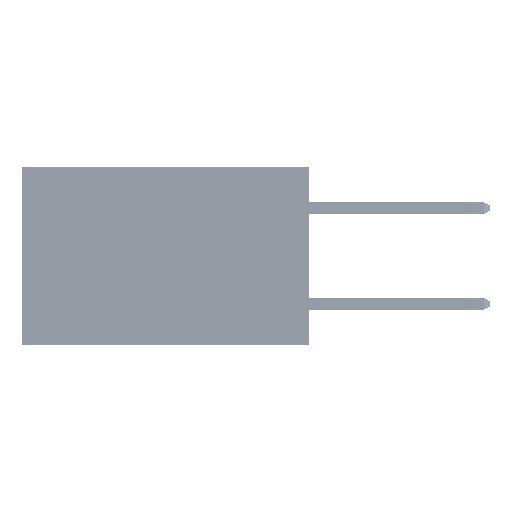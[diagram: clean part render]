
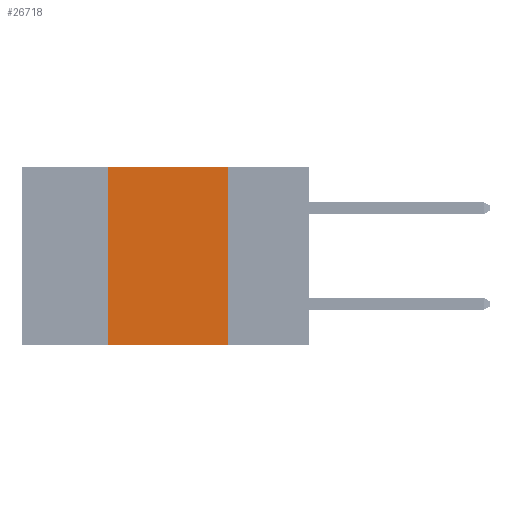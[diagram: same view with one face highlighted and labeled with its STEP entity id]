
A CAD part, left-side view. The second image highlights one B-rep face of the part: STEP entity #26718.
In plain terms, the highlighted planar face has unit normal (-1, 0, 0).
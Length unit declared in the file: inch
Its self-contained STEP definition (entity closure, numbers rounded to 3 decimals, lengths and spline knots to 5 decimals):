
#3771 = LINE ( 'NONE', #43292, #22693 ) ;
#4714 = ORIENTED_EDGE ( 'NONE', *, *, #41094, .F. ) ;
#6899 = CARTESIAN_POINT ( 'NONE',  ( 0., 0.6, 0. ) ) ;
#7054 = CARTESIAN_POINT ( 'NONE',  ( 0., 0.42, 0. ) ) ;
#7142 = EDGE_CURVE ( 'NONE', #38071, #16841, #40286, .T. ) ;
#8549 = LINE ( 'NONE', #7054, #18043 ) ;
#9423 = EDGE_CURVE ( 'NONE', #12495, #20548, #3771, .T. ) ;
#10263 = EDGE_CURVE ( 'NONE', #16841, #20548, #38269, .T. ) ;
#10936 = DIRECTION ( 'NONE',  ( 0., 0., -1. ) ) ;
#12495 = VERTEX_POINT ( 'NONE', #46830 ) ;
#15888 = EDGE_LOOP ( 'NONE', ( #47337, #34877, #4714, #20525 ) ) ;
#16715 = CARTESIAN_POINT ( 'NONE',  ( 0., 0.17, -0.37 ) ) ;
#16841 = VERTEX_POINT ( 'NONE', #40155 ) ;
#18043 = VECTOR ( 'NONE', #43375, 39.37008 ) ;
#20065 = FACE_OUTER_BOUND ( 'NONE', #15888, .T. ) ;
#20525 = ORIENTED_EDGE ( 'NONE', *, *, #9423, .T. ) ;
#20548 = VERTEX_POINT ( 'NONE', #16715 ) ;
#21169 = CARTESIAN_POINT ( 'NONE',  ( 0., 0.17, 0. ) ) ;
#22693 = VECTOR ( 'NONE', #23368, 39.37008 ) ;
#23368 = DIRECTION ( 'NONE',  ( 0., -1., 0. ) ) ;
#25179 = DIRECTION ( 'NONE',  ( 0., 0., -1. ) ) ;
#26718 = ADVANCED_FACE ( 'NONE', ( #20065 ), #42875, .F. ) ;
#29166 = DIRECTION ( 'NONE',  ( 0., -1., 0. ) ) ;
#30479 = AXIS2_PLACEMENT_3D ( 'NONE', #6899, #35032, #10936 ) ;
#34877 = ORIENTED_EDGE ( 'NONE', *, *, #7142, .F. ) ;
#35032 = DIRECTION ( 'NONE',  ( 1., 0., 0. ) ) ;
#35785 = CARTESIAN_POINT ( 'NONE',  ( 0., 0.42, 0. ) ) ;
#37003 = VECTOR ( 'NONE', #25179, 39.37008 ) ;
#37220 = CARTESIAN_POINT ( 'NONE',  ( 0., 0.6, 0. ) ) ;
#38071 = VERTEX_POINT ( 'NONE', #35785 ) ;
#38269 = LINE ( 'NONE', #21169, #37003 ) ;
#40155 = CARTESIAN_POINT ( 'NONE',  ( 0., 0.17, 0. ) ) ;
#40286 = LINE ( 'NONE', #37220, #49620 ) ;
#41094 = EDGE_CURVE ( 'NONE', #12495, #38071, #8549, .T. ) ;
#42875 = PLANE ( 'NONE',  #30479 ) ;
#43292 = CARTESIAN_POINT ( 'NONE',  ( 0., 0.6, -0.37 ) ) ;
#43375 = DIRECTION ( 'NONE',  ( 0., 0., 1. ) ) ;
#46830 = CARTESIAN_POINT ( 'NONE',  ( 0., 0.42, -0.37 ) ) ;
#47337 = ORIENTED_EDGE ( 'NONE', *, *, #10263, .F. ) ;
#49620 = VECTOR ( 'NONE', #29166, 39.37008 ) ;
